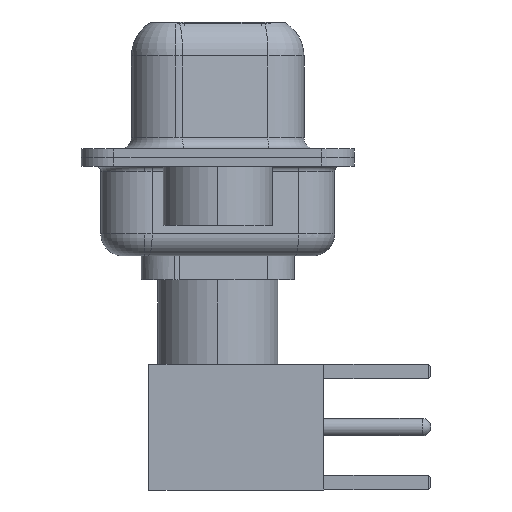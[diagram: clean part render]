
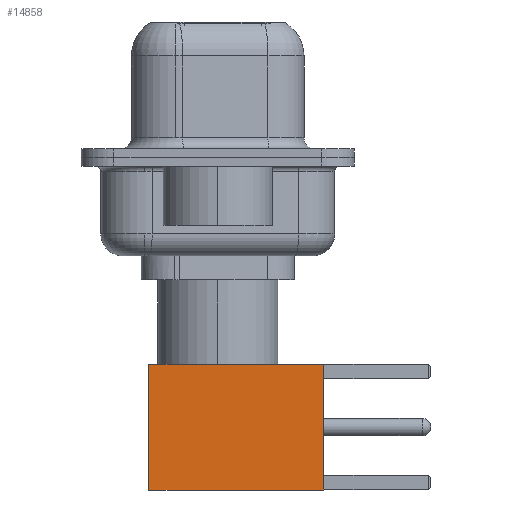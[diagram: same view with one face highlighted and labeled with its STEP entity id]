
A CAD part, left-side view. The second image highlights one B-rep face of the part: STEP entity #14858.
In plain terms, the highlighted face is planar.
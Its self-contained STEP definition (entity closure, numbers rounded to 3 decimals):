
#452 = VERTEX_POINT ( 'NONE', #14769 ) ;
#931 = AXIS2_PLACEMENT_3D ( 'NONE', #11285, #15704, #12882 ) ;
#1090 = ORIENTED_EDGE ( 'NONE', *, *, #4998, .F. ) ;
#1119 = CARTESIAN_POINT ( 'NONE',  ( -2.875, 2.875, 8. ) ) ;
#1531 = DIRECTION ( 'NONE',  ( 0., 0., -1. ) ) ;
#3250 = CARTESIAN_POINT ( 'NONE',  ( 0., 2.875, 0. ) ) ;
#4157 = ORIENTED_EDGE ( 'NONE', *, *, #16950, .T. ) ;
#4305 = CARTESIAN_POINT ( 'NONE',  ( 2.875, 2.875, 0. ) ) ;
#4998 = EDGE_CURVE ( 'NONE', #12813, #13187, #9191, .T. ) ;
#5117 = LINE ( 'NONE', #12692, #15508 ) ;
#5563 = PLANE ( 'NONE',  #931 ) ;
#5865 = LINE ( 'NONE', #3250, #15219 ) ;
#7100 = EDGE_LOOP ( 'NONE', ( #4157, #15803, #15886, #1090 ) ) ;
#7797 = DIRECTION ( 'NONE',  ( -1., 0., 0. ) ) ;
#7883 = VECTOR ( 'NONE', #10004, 1000. ) ;
#7987 = CARTESIAN_POINT ( 'NONE',  ( 0., 2.875, 8. ) ) ;
#9191 = LINE ( 'NONE', #7987, #14213 ) ;
#10004 = DIRECTION ( 'NONE',  ( 0., 0., -1. ) ) ;
#10301 = EDGE_CURVE ( 'NONE', #452, #11321, #5865, .T. ) ;
#11285 = CARTESIAN_POINT ( 'NONE',  ( 2.875, 2.875, 0. ) ) ;
#11321 = VERTEX_POINT ( 'NONE', #13125 ) ;
#12126 = EDGE_CURVE ( 'NONE', #13187, #11321, #5117, .T. ) ;
#12692 = CARTESIAN_POINT ( 'NONE',  ( -2.875, 2.875, 0. ) ) ;
#12813 = VERTEX_POINT ( 'NONE', #14736 ) ;
#12882 = DIRECTION ( 'NONE',  ( 0., 0., 1. ) ) ;
#13125 = CARTESIAN_POINT ( 'NONE',  ( -2.875, 2.875, 0. ) ) ;
#13187 = VERTEX_POINT ( 'NONE', #1119 ) ;
#14109 = FACE_OUTER_BOUND ( 'NONE', #7100, .T. ) ;
#14213 = VECTOR ( 'NONE', #7797, 1000. ) ;
#14736 = CARTESIAN_POINT ( 'NONE',  ( 2.875, 2.875, 8. ) ) ;
#14769 = CARTESIAN_POINT ( 'NONE',  ( 2.875, 2.875, 0. ) ) ;
#14858 = ADVANCED_FACE ( 'NONE', ( #14109 ), #5563, .T. ) ;
#15219 = VECTOR ( 'NONE', #15907, 1000. ) ;
#15508 = VECTOR ( 'NONE', #1531, 1000. ) ;
#15704 = DIRECTION ( 'NONE',  ( 0., 1., 0. ) ) ;
#15803 = ORIENTED_EDGE ( 'NONE', *, *, #10301, .T. ) ;
#15886 = ORIENTED_EDGE ( 'NONE', *, *, #12126, .F. ) ;
#15907 = DIRECTION ( 'NONE',  ( -1., 0., 0. ) ) ;
#16102 = LINE ( 'NONE', #4305, #7883 ) ;
#16950 = EDGE_CURVE ( 'NONE', #12813, #452, #16102, .T. ) ;
